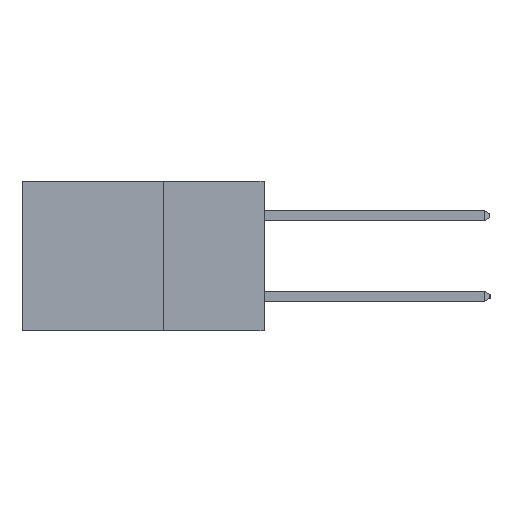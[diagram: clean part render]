
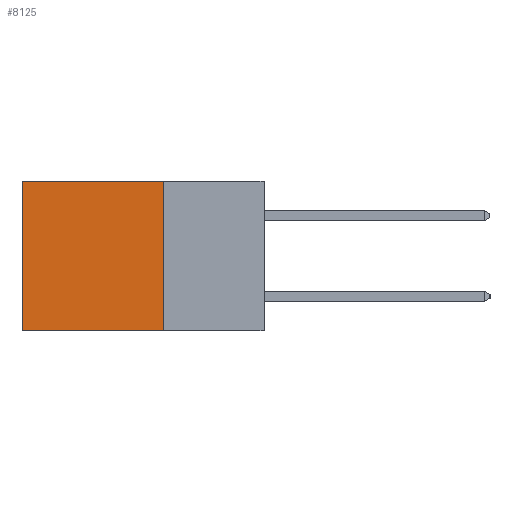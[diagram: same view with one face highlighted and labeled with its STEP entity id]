
A CAD part, left-side view. The second image highlights one B-rep face of the part: STEP entity #8125.
In plain terms, the highlighted planar face has unit normal (-1, 0, 0).
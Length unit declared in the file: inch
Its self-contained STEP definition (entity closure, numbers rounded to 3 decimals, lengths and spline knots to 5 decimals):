
#1518 = VERTEX_POINT ( 'NONE', #3446 ) ;
#1677 = VERTEX_POINT ( 'NONE', #4458 ) ;
#1773 = ORIENTED_EDGE ( 'NONE', *, *, #15774, .T. ) ;
#1793 = LINE ( 'NONE', #8884, #7792 ) ;
#2723 = VERTEX_POINT ( 'NONE', #5996 ) ;
#3446 = CARTESIAN_POINT ( 'NONE',  ( 0.2615, 0.25, 0. ) ) ;
#4458 = CARTESIAN_POINT ( 'NONE',  ( 0.2615, 0.25, -0.37 ) ) ;
#4620 = DIRECTION ( 'NONE',  ( 0., 1., 0. ) ) ;
#4747 = EDGE_CURVE ( 'NONE', #1677, #12432, #15211, .T. ) ;
#5003 = CARTESIAN_POINT ( 'NONE',  ( 0.2615, 0.25, -0.37 ) ) ;
#5035 = ORIENTED_EDGE ( 'NONE', *, *, #8977, .T. ) ;
#5996 = CARTESIAN_POINT ( 'NONE',  ( 0.2615, 0.6, 0. ) ) ;
#6141 = LINE ( 'NONE', #6690, #9120 ) ;
#6507 = CARTESIAN_POINT ( 'NONE',  ( 0.2615, 0.6, -0.37 ) ) ;
#6690 = CARTESIAN_POINT ( 'NONE',  ( 0.2615, 0.25, -0.37 ) ) ;
#6723 = DIRECTION ( 'NONE',  ( 0., 0., -1. ) ) ;
#6995 = FACE_OUTER_BOUND ( 'NONE', #13447, .T. ) ;
#7575 = DIRECTION ( 'NONE',  ( 0., 1., 0. ) ) ;
#7792 = VECTOR ( 'NONE', #7575, 39.37008 ) ;
#7867 = ORIENTED_EDGE ( 'NONE', *, *, #10790, .F. ) ;
#7962 = VECTOR ( 'NONE', #9011, 39.37008 ) ;
#8125 = ADVANCED_FACE ( 'NONE', ( #6995 ), #14151, .F. ) ;
#8884 = CARTESIAN_POINT ( 'NONE',  ( 0.2615, 0.25, 0. ) ) ;
#8977 = EDGE_CURVE ( 'NONE', #1518, #2723, #1793, .T. ) ;
#9011 = DIRECTION ( 'NONE',  ( 0., 0., -1. ) ) ;
#9120 = VECTOR ( 'NONE', #6723, 39.37008 ) ;
#10790 = EDGE_CURVE ( 'NONE', #1518, #1677, #6141, .T. ) ;
#11571 = AXIS2_PLACEMENT_3D ( 'NONE', #13600, #13464, #13421 ) ;
#12432 = VERTEX_POINT ( 'NONE', #14096 ) ;
#13421 = DIRECTION ( 'NONE',  ( 0., 0., -1. ) ) ;
#13447 = EDGE_LOOP ( 'NONE', ( #1773, #13612, #7867, #5035 ) ) ;
#13464 = DIRECTION ( 'NONE',  ( 1., 0., 0. ) ) ;
#13600 = CARTESIAN_POINT ( 'NONE',  ( 0.2615, 0.25, -0.37 ) ) ;
#13612 = ORIENTED_EDGE ( 'NONE', *, *, #4747, .F. ) ;
#14016 = LINE ( 'NONE', #6507, #7962 ) ;
#14096 = CARTESIAN_POINT ( 'NONE',  ( 0.2615, 0.6, -0.37 ) ) ;
#14143 = VECTOR ( 'NONE', #4620, 39.37008 ) ;
#14151 = PLANE ( 'NONE',  #11571 ) ;
#15211 = LINE ( 'NONE', #5003, #14143 ) ;
#15774 = EDGE_CURVE ( 'NONE', #2723, #12432, #14016, .T. ) ;
